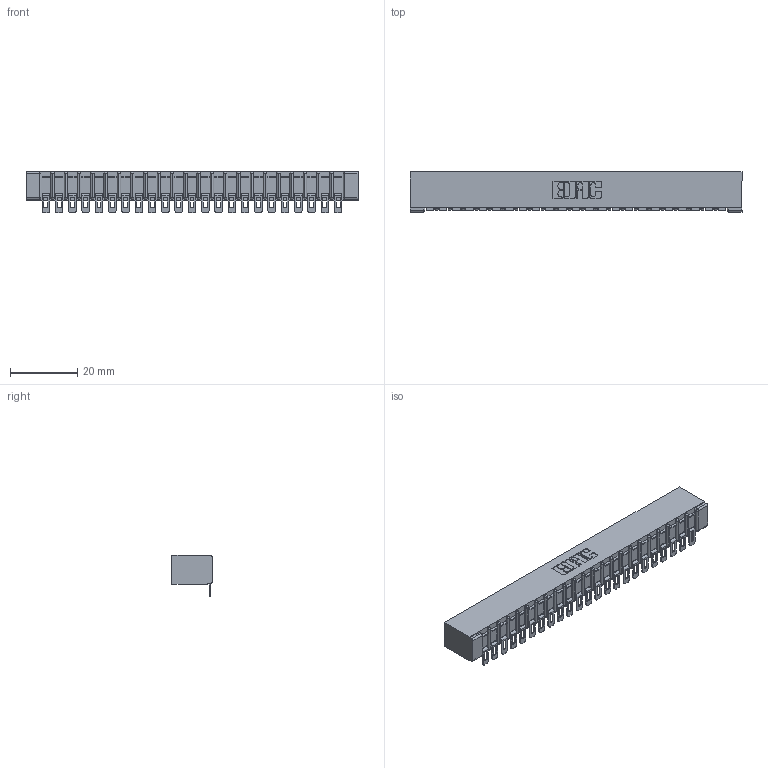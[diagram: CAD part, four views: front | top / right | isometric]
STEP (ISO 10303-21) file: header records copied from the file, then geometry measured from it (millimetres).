
FILE_DESCRIPTION (( 'STEP AP203' ), '1' );
FILE_NAME ('307-023-454-101.STEP', '2020-09-27T09:24:13', ( '' ), ( '' ), 'SwSTEP 2.0', 'SolidWorks 2020', '' );
FILE_SCHEMA (( 'CONFIG_CONTROL_DESIGN' ));
Length unit declared in the file: inch
Products named in the file (3): 307-290-002_554; 307 Part_No Mounting Lugs; 307-023-454-101
Assembly tree (24 placements, depth 2):
  307-023-454-101
    307 Part_No Mounting Lugs
    307-290-002_554  x23
Bounding box: 99.01 x 12.01 x 12.52 mm (x, y, z)
Volume: 6787.5 mm3; surface area: 13002.8 mm2
Topology: 24 solids, 24 shells, 1997 faces, 6118 edges, 4012 vertices
Faces by surface type: plane 1124, cylinder 825, sphere 48
Entity records: 22747 total; most frequent: CARTESIAN_POINT 3834, ORIENTED_EDGE 3824, DIRECTION 3738, EDGE_CURVE 1912, VECTOR 1450, LINE 1450, VERTEX_POINT 1240, AXIS2_PLACEMENT_3D 1144
